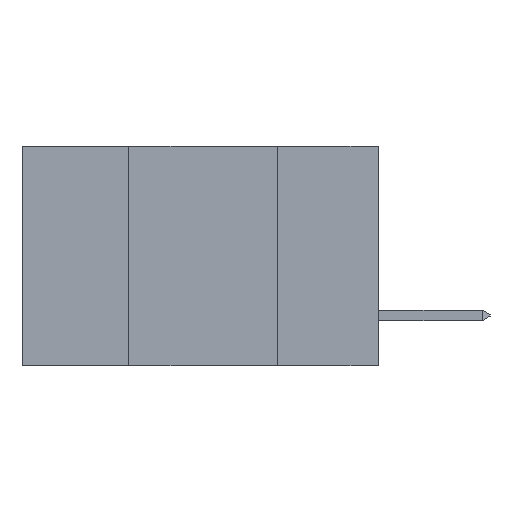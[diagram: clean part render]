
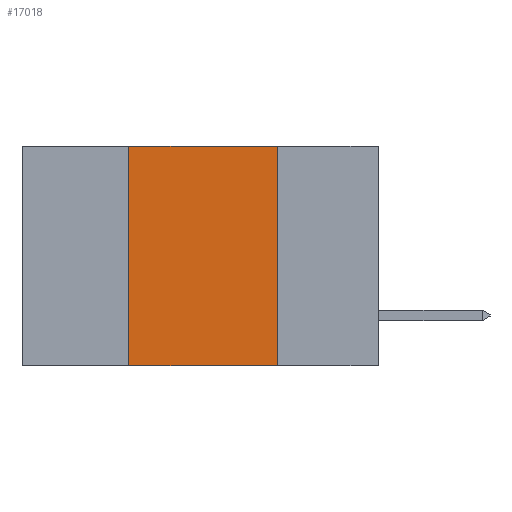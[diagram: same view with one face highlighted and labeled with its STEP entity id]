
A CAD part, left-side view. The second image highlights one B-rep face of the part: STEP entity #17018.
In plain terms, the highlighted planar face has unit normal (-1, 0, 0).
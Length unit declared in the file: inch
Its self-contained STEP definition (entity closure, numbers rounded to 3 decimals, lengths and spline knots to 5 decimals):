
#15 = CARTESIAN_POINT ( 'NONE',  ( 0., 0.42, -0.37 ) ) ;
#17 = DIRECTION ( 'NONE',  ( 0., 0., -1. ) ) ;
#1069 = DIRECTION ( 'NONE',  ( 0., -1., 0. ) ) ;
#1188 = CARTESIAN_POINT ( 'NONE',  ( 0., 0.6, 0. ) ) ;
#1642 = VECTOR ( 'NONE', #5878, 39.37008 ) ;
#2133 = LINE ( 'NONE', #4288, #1642 ) ;
#2799 = VERTEX_POINT ( 'NONE', #16937 ) ;
#2962 = ORIENTED_EDGE ( 'NONE', *, *, #7120, .F. ) ;
#3007 = CARTESIAN_POINT ( 'NONE',  ( 0., 0.17, -0.37 ) ) ;
#3234 = ORIENTED_EDGE ( 'NONE', *, *, #8139, .F. ) ;
#3601 = VECTOR ( 'NONE', #13073, 39.37008 ) ;
#3913 = VECTOR ( 'NONE', #1069, 39.37008 ) ;
#3946 = VERTEX_POINT ( 'NONE', #12291 ) ;
#4112 = LINE ( 'NONE', #12941, #3601 ) ;
#4288 = CARTESIAN_POINT ( 'NONE',  ( 0., 0.17, -0.37 ) ) ;
#5878 = DIRECTION ( 'NONE',  ( 0., 0., -1. ) ) ;
#7120 = EDGE_CURVE ( 'NONE', #3946, #14101, #16089, .T. ) ;
#7322 = ORIENTED_EDGE ( 'NONE', *, *, #15504, .F. ) ;
#7790 = CARTESIAN_POINT ( 'NONE',  ( 0., 0.6, 0. ) ) ;
#8139 = EDGE_CURVE ( 'NONE', #2799, #3946, #11615, .T. ) ;
#9178 = EDGE_CURVE ( 'NONE', #2799, #12967, #4112, .T. ) ;
#9354 = DIRECTION ( 'NONE',  ( 1., 0., 0. ) ) ;
#11615 = LINE ( 'NONE', #15, #19049 ) ;
#12291 = CARTESIAN_POINT ( 'NONE',  ( 0., 0.42, 0. ) ) ;
#12941 = CARTESIAN_POINT ( 'NONE',  ( 0., 0.6, -0.37 ) ) ;
#12967 = VERTEX_POINT ( 'NONE', #3007 ) ;
#13073 = DIRECTION ( 'NONE',  ( 0., -1., 0. ) ) ;
#14101 = VERTEX_POINT ( 'NONE', #18884 ) ;
#14415 = ORIENTED_EDGE ( 'NONE', *, *, #9178, .T. ) ;
#15504 = EDGE_CURVE ( 'NONE', #14101, #12967, #2133, .T. ) ;
#16087 = AXIS2_PLACEMENT_3D ( 'NONE', #7790, #9354, #17 ) ;
#16089 = LINE ( 'NONE', #1188, #3913 ) ;
#16718 = FACE_OUTER_BOUND ( 'NONE', #18664, .T. ) ;
#16937 = CARTESIAN_POINT ( 'NONE',  ( 0., 0.42, -0.37 ) ) ;
#17018 = ADVANCED_FACE ( 'NONE', ( #16718 ), #18357, .F. ) ;
#18357 = PLANE ( 'NONE',  #16087 ) ;
#18664 = EDGE_LOOP ( 'NONE', ( #7322, #2962, #3234, #14415 ) ) ;
#18884 = CARTESIAN_POINT ( 'NONE',  ( 0., 0.17, 0. ) ) ;
#19049 = VECTOR ( 'NONE', #19530, 39.37008 ) ;
#19530 = DIRECTION ( 'NONE',  ( 0., 0., 1. ) ) ;
